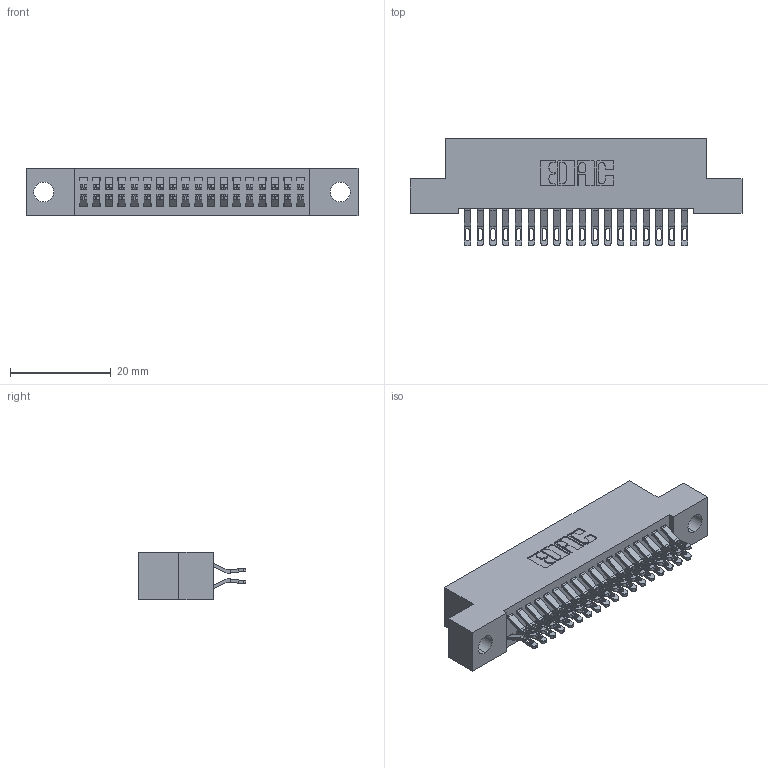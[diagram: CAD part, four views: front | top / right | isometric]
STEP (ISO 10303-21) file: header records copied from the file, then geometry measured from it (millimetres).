
FILE_DESCRIPTION (( 'STEP AP203' ), '1' );
FILE_NAME ('392-036-555-204.STEP', '2019-10-07T17:31:29', ( '' ), ( '' ), 'SwSTEP 2.0', 'SolidWorks 2016', '' );
FILE_SCHEMA (( 'CONFIG_CONTROL_DESIGN' ));
Length unit declared in the file: inch
Products named in the file (3): 342 Part_.156 TH; 345-292-001_555 Tail; 392-036-555-204
Assembly tree (37 placements, depth 2):
  392-036-555-204
    342 Part_.156 TH
    345-292-001_555 Tail  x36
Bounding box: 66.04 x 21.47 x 9.4 mm (x, y, z)
Volume: 5833.1 mm3; surface area: 9076 mm2
Topology: 37 solids, 37 shells, 2198 faces, 6887 edges, 4590 vertices
Faces by surface type: plane 1290, cylinder 908
Entity records: 14881 total; most frequent: CARTESIAN_POINT 2528, ORIENTED_EDGE 2434, DIRECTION 2173, EDGE_CURVE 1217, VECTOR 1069, LINE 1069, VERTEX_POINT 810, AXIS2_PLACEMENT_3D 552
